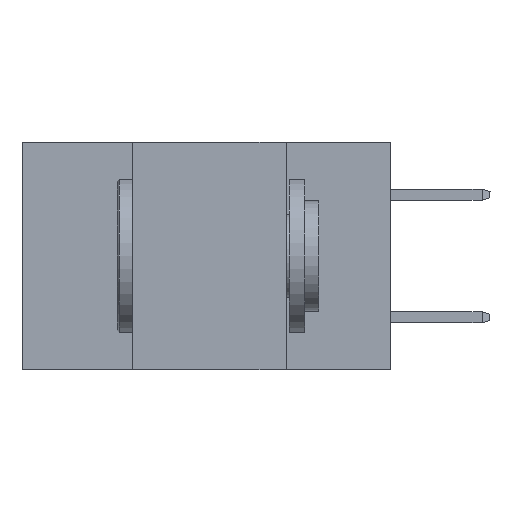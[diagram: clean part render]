
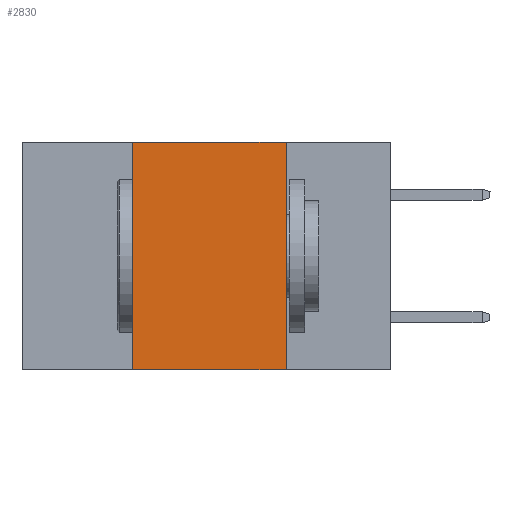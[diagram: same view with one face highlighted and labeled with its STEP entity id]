
A CAD part, left-side view. The second image highlights one B-rep face of the part: STEP entity #2830.
In plain terms, the highlighted planar face has unit normal (-1, 0, 0).
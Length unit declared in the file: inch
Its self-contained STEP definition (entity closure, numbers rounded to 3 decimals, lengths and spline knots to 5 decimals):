
#217 = EDGE_CURVE ( 'NONE', #8344, #4151, #7936, .T. ) ;
#636 = EDGE_CURVE ( 'NONE', #6867, #4151, #5611, .T. ) ;
#787 = EDGE_LOOP ( 'NONE', ( #7677, #9090, #11978, #14127 ) ) ;
#953 = DIRECTION ( 'NONE',  ( 0., 0., -1. ) ) ;
#1326 = CARTESIAN_POINT ( 'NONE',  ( 0., 0.6, -0.37 ) ) ;
#1812 = VECTOR ( 'NONE', #9552, 39.37008 ) ;
#2323 = CARTESIAN_POINT ( 'NONE',  ( 0., 0.17, 0. ) ) ;
#2646 = FACE_OUTER_BOUND ( 'NONE', #787, .T. ) ;
#2830 = ADVANCED_FACE ( 'NONE', ( #2646 ), #6444, .F. ) ;
#3385 = DIRECTION ( 'NONE',  ( 0., 0., 1. ) ) ;
#3426 = CARTESIAN_POINT ( 'NONE',  ( 0., 0.17, -0.37 ) ) ;
#3992 = AXIS2_PLACEMENT_3D ( 'NONE', #8760, #11237, #953 ) ;
#4151 = VERTEX_POINT ( 'NONE', #3426 ) ;
#4971 = VERTEX_POINT ( 'NONE', #9634 ) ;
#5326 = LINE ( 'NONE', #9825, #12932 ) ;
#5544 = DIRECTION ( 'NONE',  ( 0., 0., -1. ) ) ;
#5611 = LINE ( 'NONE', #12568, #7940 ) ;
#6255 = LINE ( 'NONE', #13030, #14956 ) ;
#6444 = PLANE ( 'NONE',  #3992 ) ;
#6867 = VERTEX_POINT ( 'NONE', #2323 ) ;
#7677 = ORIENTED_EDGE ( 'NONE', *, *, #636, .F. ) ;
#7833 = EDGE_CURVE ( 'NONE', #4971, #6867, #6255, .T. ) ;
#7936 = LINE ( 'NONE', #1326, #1812 ) ;
#7940 = VECTOR ( 'NONE', #5544, 39.37008 ) ;
#8344 = VERTEX_POINT ( 'NONE', #9711 ) ;
#8760 = CARTESIAN_POINT ( 'NONE',  ( 0., 0.6, 0. ) ) ;
#9090 = ORIENTED_EDGE ( 'NONE', *, *, #7833, .F. ) ;
#9552 = DIRECTION ( 'NONE',  ( 0., -1., 0. ) ) ;
#9634 = CARTESIAN_POINT ( 'NONE',  ( 0., 0.42, 0. ) ) ;
#9711 = CARTESIAN_POINT ( 'NONE',  ( 0., 0.42, -0.37 ) ) ;
#9825 = CARTESIAN_POINT ( 'NONE',  ( 0., 0.42, 0. ) ) ;
#11237 = DIRECTION ( 'NONE',  ( 1., 0., 0. ) ) ;
#11693 = EDGE_CURVE ( 'NONE', #8344, #4971, #5326, .T. ) ;
#11978 = ORIENTED_EDGE ( 'NONE', *, *, #11693, .F. ) ;
#12568 = CARTESIAN_POINT ( 'NONE',  ( 0., 0.17, 0. ) ) ;
#12932 = VECTOR ( 'NONE', #3385, 39.37008 ) ;
#13030 = CARTESIAN_POINT ( 'NONE',  ( 0., 0.6, 0. ) ) ;
#13080 = DIRECTION ( 'NONE',  ( 0., -1., 0. ) ) ;
#14127 = ORIENTED_EDGE ( 'NONE', *, *, #217, .T. ) ;
#14956 = VECTOR ( 'NONE', #13080, 39.37008 ) ;
